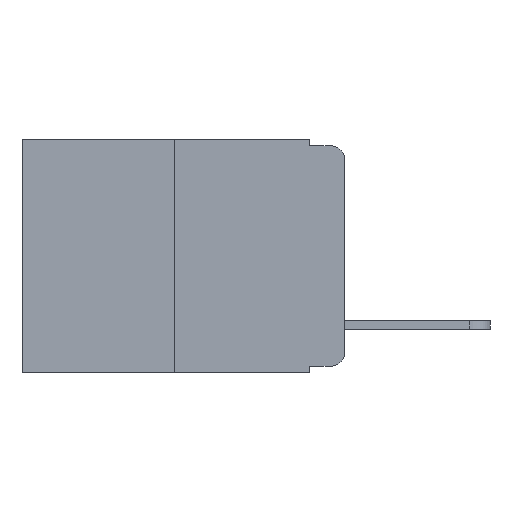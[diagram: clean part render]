
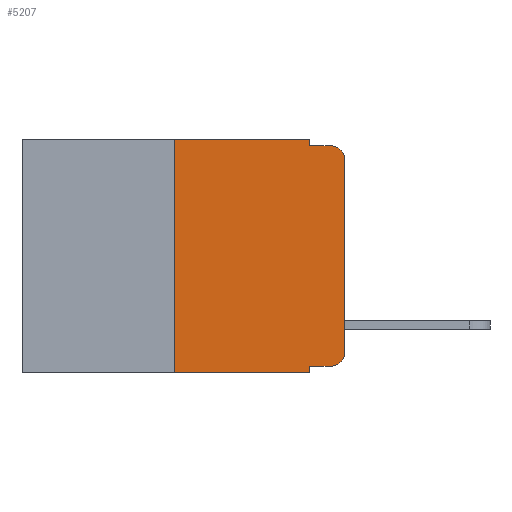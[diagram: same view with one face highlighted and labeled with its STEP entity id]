
A CAD part, left-side view. The second image highlights one B-rep face of the part: STEP entity #5207.
In plain terms, the highlighted planar face has unit normal (-1, 0, 0).
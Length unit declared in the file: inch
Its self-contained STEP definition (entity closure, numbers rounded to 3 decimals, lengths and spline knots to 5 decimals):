
#404 = LINE ( 'NONE', #12300, #10963 ) ;
#896 = LINE ( 'NONE', #8416, #6055 ) ;
#1100 = FACE_OUTER_BOUND ( 'NONE', #1447, .T. ) ;
#1206 = VERTEX_POINT ( 'NONE', #1345 ) ;
#1335 = VERTEX_POINT ( 'NONE', #6549 ) ;
#1336 = EDGE_CURVE ( 'NONE', #6383, #2691, #1879, .T. ) ;
#1345 = CARTESIAN_POINT ( 'NONE',  ( 0., 0.02, -0.01 ) ) ;
#1437 = VERTEX_POINT ( 'NONE', #5415 ) ;
#1447 = EDGE_LOOP ( 'NONE', ( #4654, #4703, #7794, #4450, #7704, #7976, #7368, #7437, #6121, #6510 ) ) ;
#1564 = VECTOR ( 'NONE', #2072, 39.37008 ) ;
#1879 = CIRCLE ( 'NONE', #12566, 0.02 ) ;
#2072 = DIRECTION ( 'NONE',  ( 0., 0., -1. ) ) ;
#2235 = DIRECTION ( 'NONE',  ( 0., 0., 1. ) ) ;
#2337 = DIRECTION ( 'NONE',  ( 1., 0., 0. ) ) ;
#2385 = EDGE_CURVE ( 'NONE', #1437, #6009, #896, .T. ) ;
#2430 = CARTESIAN_POINT ( 'NONE',  ( 0., 0.051, -0.343 ) ) ;
#2691 = VERTEX_POINT ( 'NONE', #11222 ) ;
#2746 = CARTESIAN_POINT ( 'NONE',  ( 0., 0.25, 0. ) ) ;
#2793 = DIRECTION ( 'NONE',  ( 0., 0., -1. ) ) ;
#2807 = DIRECTION ( 'NONE',  ( -1., 0., 0. ) ) ;
#2828 = CARTESIAN_POINT ( 'NONE',  ( 0., 0.02, -0.03 ) ) ;
#3166 = LINE ( 'NONE', #3860, #1564 ) ;
#3470 = EDGE_CURVE ( 'NONE', #12767, #6009, #6183, .T. ) ;
#3860 = CARTESIAN_POINT ( 'NONE',  ( 0., 0.051, 0. ) ) ;
#4170 = DIRECTION ( 'NONE',  ( 0., 0., 1. ) ) ;
#4231 = CARTESIAN_POINT ( 'NONE',  ( 0., 0., 0. ) ) ;
#4441 = EDGE_CURVE ( 'NONE', #8742, #11603, #3166, .T. ) ;
#4450 = ORIENTED_EDGE ( 'NONE', *, *, #4441, .F. ) ;
#4654 = ORIENTED_EDGE ( 'NONE', *, *, #11700, .T. ) ;
#4703 = ORIENTED_EDGE ( 'NONE', *, *, #9255, .T. ) ;
#5074 = CARTESIAN_POINT ( 'NONE',  ( 0., 0.02, -0.313 ) ) ;
#5110 = LINE ( 'NONE', #12760, #9965 ) ;
#5207 = ADVANCED_FACE ( 'NONE', ( #1100 ), #12535, .F. ) ;
#5232 = VECTOR ( 'NONE', #6829, 39.37008 ) ;
#5237 = VECTOR ( 'NONE', #2235, 39.37008 ) ;
#5249 = CARTESIAN_POINT ( 'NONE',  ( 0., 0.25, -0.343 ) ) ;
#5274 = AXIS2_PLACEMENT_3D ( 'NONE', #2828, #2807, #2793 ) ;
#5415 = CARTESIAN_POINT ( 'NONE',  ( 0., 0.051, -0.333 ) ) ;
#5595 = CARTESIAN_POINT ( 'NONE',  ( 0., 0.051, -0.01 ) ) ;
#5929 = LINE ( 'NONE', #2746, #5237 ) ;
#6009 = VERTEX_POINT ( 'NONE', #2430 ) ;
#6055 = VECTOR ( 'NONE', #6518, 39.37008 ) ;
#6072 = DIRECTION ( 'NONE',  ( 0., 0., -1. ) ) ;
#6121 = ORIENTED_EDGE ( 'NONE', *, *, #11079, .T. ) ;
#6183 = LINE ( 'NONE', #6900, #5232 ) ;
#6383 = VERTEX_POINT ( 'NONE', #9019 ) ;
#6510 = ORIENTED_EDGE ( 'NONE', *, *, #1336, .T. ) ;
#6518 = DIRECTION ( 'NONE',  ( 0., 0., -1. ) ) ;
#6549 = CARTESIAN_POINT ( 'NONE',  ( 0., 0., -0.03 ) ) ;
#6744 = VECTOR ( 'NONE', #11140, 39.37008 ) ;
#6829 = DIRECTION ( 'NONE',  ( 0., -1., 0. ) ) ;
#6900 = CARTESIAN_POINT ( 'NONE',  ( 0., 0.473, -0.343 ) ) ;
#7221 = DIRECTION ( 'NONE',  ( -1., 0., 0. ) ) ;
#7277 = CIRCLE ( 'NONE', #5274, 0.02 ) ;
#7368 = ORIENTED_EDGE ( 'NONE', *, *, #3470, .T. ) ;
#7437 = ORIENTED_EDGE ( 'NONE', *, *, #2385, .F. ) ;
#7704 = ORIENTED_EDGE ( 'NONE', *, *, #11016, .F. ) ;
#7794 = ORIENTED_EDGE ( 'NONE', *, *, #11176, .F. ) ;
#7976 = ORIENTED_EDGE ( 'NONE', *, *, #11785, .F. ) ;
#8083 = VERTEX_POINT ( 'NONE', #12194 ) ;
#8416 = CARTESIAN_POINT ( 'NONE',  ( 0., 0.051, 0. ) ) ;
#8568 = AXIS2_PLACEMENT_3D ( 'NONE', #12786, #2337, #10117 ) ;
#8742 = VERTEX_POINT ( 'NONE', #10373 ) ;
#9019 = CARTESIAN_POINT ( 'NONE',  ( 0., 0.02, -0.333 ) ) ;
#9255 = EDGE_CURVE ( 'NONE', #1335, #1206, #7277, .T. ) ;
#9318 = LINE ( 'NONE', #11218, #6744 ) ;
#9965 = VECTOR ( 'NONE', #12748, 39.37008 ) ;
#10117 = DIRECTION ( 'NONE',  ( 0., 0., -1. ) ) ;
#10199 = LINE ( 'NONE', #4231, #12278 ) ;
#10373 = CARTESIAN_POINT ( 'NONE',  ( 0., 0.051, 0. ) ) ;
#10963 = VECTOR ( 'NONE', #12185, 39.37008 ) ;
#11016 = EDGE_CURVE ( 'NONE', #8083, #8742, #5110, .T. ) ;
#11079 = EDGE_CURVE ( 'NONE', #1437, #6383, #404, .T. ) ;
#11140 = DIRECTION ( 'NONE',  ( 0., -1., 0. ) ) ;
#11176 = EDGE_CURVE ( 'NONE', #11603, #1206, #9318, .T. ) ;
#11218 = CARTESIAN_POINT ( 'NONE',  ( 0., 0.051, -0.01 ) ) ;
#11222 = CARTESIAN_POINT ( 'NONE',  ( 0., 0., -0.313 ) ) ;
#11603 = VERTEX_POINT ( 'NONE', #5595 ) ;
#11700 = EDGE_CURVE ( 'NONE', #2691, #1335, #10199, .T. ) ;
#11785 = EDGE_CURVE ( 'NONE', #12767, #8083, #5929, .T. ) ;
#12185 = DIRECTION ( 'NONE',  ( 0., -1., 0. ) ) ;
#12194 = CARTESIAN_POINT ( 'NONE',  ( 0., 0.25, 0. ) ) ;
#12278 = VECTOR ( 'NONE', #4170, 39.37008 ) ;
#12300 = CARTESIAN_POINT ( 'NONE',  ( 0., 0.051, -0.333 ) ) ;
#12535 = PLANE ( 'NONE',  #8568 ) ;
#12566 = AXIS2_PLACEMENT_3D ( 'NONE', #5074, #7221, #6072 ) ;
#12748 = DIRECTION ( 'NONE',  ( 0., -1., 0. ) ) ;
#12760 = CARTESIAN_POINT ( 'NONE',  ( 0., 0.473, 0. ) ) ;
#12767 = VERTEX_POINT ( 'NONE', #5249 ) ;
#12786 = CARTESIAN_POINT ( 'NONE',  ( 0., 0.473, 0. ) ) ;
